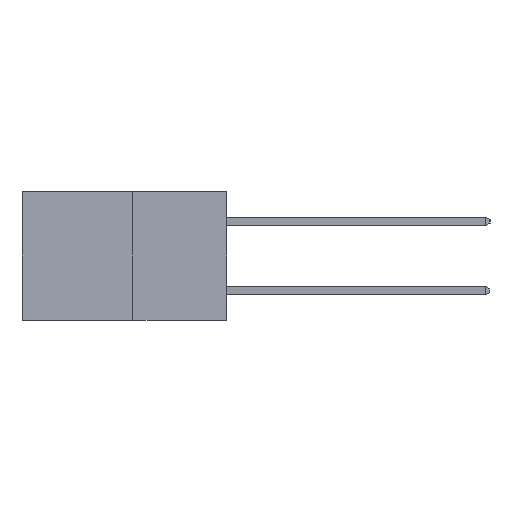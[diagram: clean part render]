
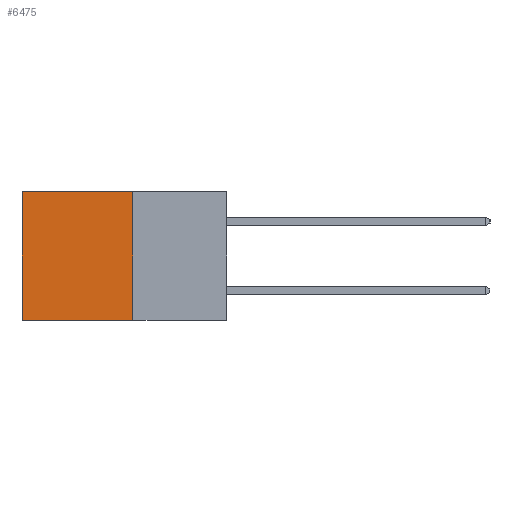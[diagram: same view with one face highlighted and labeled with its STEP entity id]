
A CAD part, left-side view. The second image highlights one B-rep face of the part: STEP entity #6475.
In plain terms, the highlighted planar face has unit normal (-1, 0, 0).
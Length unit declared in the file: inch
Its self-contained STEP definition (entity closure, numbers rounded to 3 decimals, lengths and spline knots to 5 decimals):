
#142 = VECTOR ( 'NONE', #8301, 39.37008 ) ;
#806 = LINE ( 'NONE', #9605, #9259 ) ;
#874 = LINE ( 'NONE', #11217, #8991 ) ;
#2492 = ORIENTED_EDGE ( 'NONE', *, *, #6684, .T. ) ;
#2916 = EDGE_CURVE ( 'NONE', #11862, #5391, #806, .T. ) ;
#3460 = EDGE_CURVE ( 'NONE', #5316, #7494, #5729, .T. ) ;
#4179 = ORIENTED_EDGE ( 'NONE', *, *, #2916, .T. ) ;
#4445 = EDGE_CURVE ( 'NONE', #11862, #5316, #5377, .T. ) ;
#4724 = CARTESIAN_POINT ( 'NONE',  ( 0.277, 0.27, -0.37 ) ) ;
#4811 = DIRECTION ( 'NONE',  ( 0., 0., -1. ) ) ;
#5316 = VERTEX_POINT ( 'NONE', #7499 ) ;
#5377 = LINE ( 'NONE', #4724, #8211 ) ;
#5391 = VERTEX_POINT ( 'NONE', #6833 ) ;
#5729 = LINE ( 'NONE', #8797, #142 ) ;
#6475 = ADVANCED_FACE ( 'NONE', ( #9168 ), #11172, .F. ) ;
#6684 = EDGE_CURVE ( 'NONE', #5391, #7494, #874, .T. ) ;
#6833 = CARTESIAN_POINT ( 'NONE',  ( 0.277, 0.59, 0. ) ) ;
#7234 = CARTESIAN_POINT ( 'NONE',  ( 0.277, 0.27, 0. ) ) ;
#7494 = VERTEX_POINT ( 'NONE', #12451 ) ;
#7499 = CARTESIAN_POINT ( 'NONE',  ( 0.277, 0.27, -0.37 ) ) ;
#7630 = ORIENTED_EDGE ( 'NONE', *, *, #3460, .F. ) ;
#8211 = VECTOR ( 'NONE', #4811, 39.37008 ) ;
#8281 = ORIENTED_EDGE ( 'NONE', *, *, #4445, .F. ) ;
#8301 = DIRECTION ( 'NONE',  ( 0., 1., 0. ) ) ;
#8403 = AXIS2_PLACEMENT_3D ( 'NONE', #13322, #11126, #11039 ) ;
#8731 = DIRECTION ( 'NONE',  ( 0., 1., 0. ) ) ;
#8797 = CARTESIAN_POINT ( 'NONE',  ( 0.277, 0.27, -0.37 ) ) ;
#8991 = VECTOR ( 'NONE', #12286, 39.37008 ) ;
#9168 = FACE_OUTER_BOUND ( 'NONE', #12738, .T. ) ;
#9259 = VECTOR ( 'NONE', #8731, 39.37008 ) ;
#9605 = CARTESIAN_POINT ( 'NONE',  ( 0.277, 0.27, 0. ) ) ;
#11039 = DIRECTION ( 'NONE',  ( 0., 0., -1. ) ) ;
#11126 = DIRECTION ( 'NONE',  ( 1., 0., 0. ) ) ;
#11172 = PLANE ( 'NONE',  #8403 ) ;
#11217 = CARTESIAN_POINT ( 'NONE',  ( 0.277, 0.59, -0.37 ) ) ;
#11862 = VERTEX_POINT ( 'NONE', #7234 ) ;
#12286 = DIRECTION ( 'NONE',  ( 0., 0., -1. ) ) ;
#12451 = CARTESIAN_POINT ( 'NONE',  ( 0.277, 0.59, -0.37 ) ) ;
#12738 = EDGE_LOOP ( 'NONE', ( #2492, #7630, #8281, #4179 ) ) ;
#13322 = CARTESIAN_POINT ( 'NONE',  ( 0.277, 0.27, -0.37 ) ) ;
